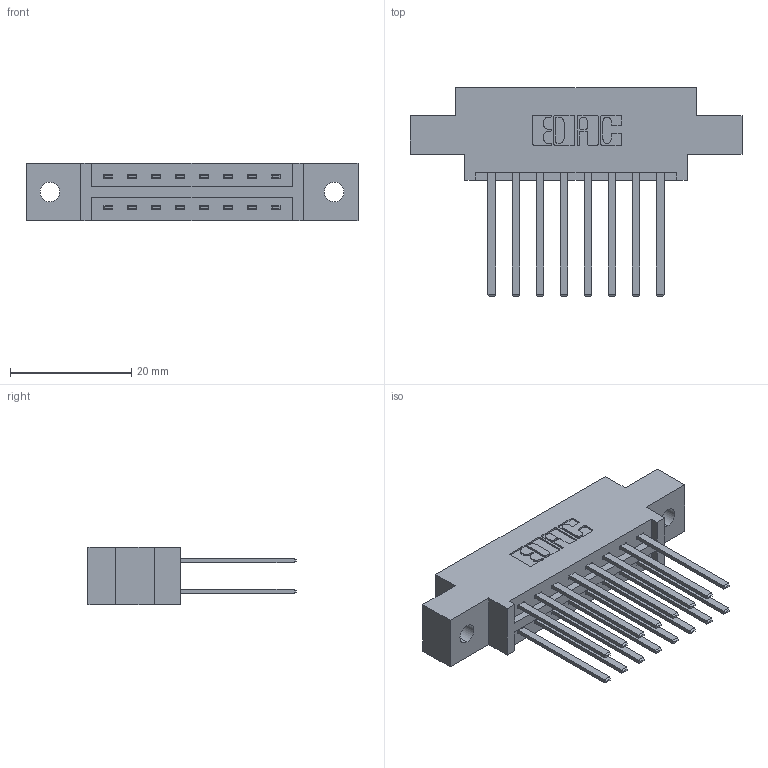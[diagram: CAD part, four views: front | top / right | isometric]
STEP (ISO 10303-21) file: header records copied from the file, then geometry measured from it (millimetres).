
FILE_DESCRIPTION (( 'STEP AP203' ), '1' );
FILE_NAME ('387-016-544-802.STEP', '2019-10-15T23:32:05', ( '' ), ( '' ), 'SwSTEP 2.0', 'SolidWorks 2016', '' );
FILE_SCHEMA (( 'CONFIG_CONTROL_DESIGN' ));
Length unit declared in the file: inch
Products named in the file (3): 387-016-544-802; 337 Part_0.170 Offset - 0.128 Dia; 345-292-001_345-293-144
Assembly tree (17 placements, depth 2):
  387-016-544-802
    337 Part_0.170 Offset - 0.128 Dia
    345-292-001_345-293-144  x16
Bounding box: 54.71 x 34.3 x 9.4 mm (x, y, z)
Volume: 5383.5 mm3; surface area: 6323.6 mm2
Topology: 17 solids, 17 shells, 886 faces, 2611 edges, 1718 vertices
Faces by surface type: plane 618, cylinder 268
Entity records: 10551 total; most frequent: CARTESIAN_POINT 1806, ORIENTED_EDGE 1742, DIRECTION 1595, EDGE_CURVE 871, LINE 747, VECTOR 747, VERTEX_POINT 578, AXIS2_PLACEMENT_3D 424
